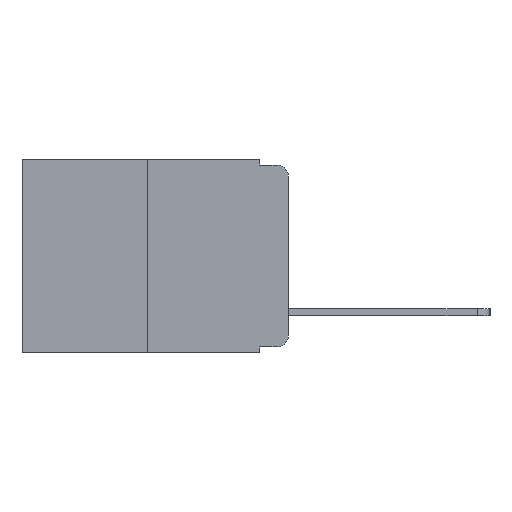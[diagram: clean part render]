
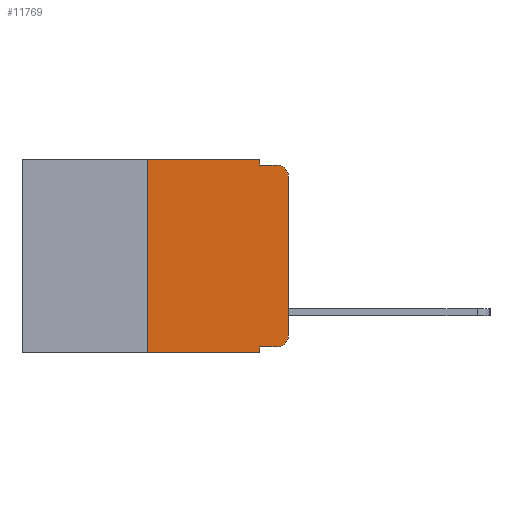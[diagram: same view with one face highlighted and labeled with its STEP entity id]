
A CAD part, left-side view. The second image highlights one B-rep face of the part: STEP entity #11769.
In plain terms, the highlighted planar face has unit normal (-1, 0, 0).
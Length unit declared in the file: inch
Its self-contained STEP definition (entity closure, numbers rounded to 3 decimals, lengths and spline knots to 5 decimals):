
#144 = ORIENTED_EDGE ( 'NONE', *, *, #9929, .F. ) ;
#289 = EDGE_CURVE ( 'NONE', #15602, #3585, #14269, .T. ) ;
#382 = CARTESIAN_POINT ( 'NONE',  ( 0., 0., 0. ) ) ;
#450 = CARTESIAN_POINT ( 'NONE',  ( 0., 0.25, 0. ) ) ;
#465 = ORIENTED_EDGE ( 'NONE', *, *, #289, .F. ) ;
#597 = EDGE_CURVE ( 'NONE', #3585, #1337, #13686, .T. ) ;
#1115 = PLANE ( 'NONE',  #10771 ) ;
#1337 = VERTEX_POINT ( 'NONE', #8802 ) ;
#1587 = EDGE_CURVE ( 'NONE', #6925, #15602, #7060, .T. ) ;
#1869 = VECTOR ( 'NONE', #12917, 39.37008 ) ;
#1883 = AXIS2_PLACEMENT_3D ( 'NONE', #12427, #4778, #13621 ) ;
#1904 = CARTESIAN_POINT ( 'NONE',  ( 0., 0.051, 0. ) ) ;
#1936 = EDGE_CURVE ( 'NONE', #15702, #2040, #3528, .T. ) ;
#2040 = VERTEX_POINT ( 'NONE', #13133 ) ;
#2333 = ORIENTED_EDGE ( 'NONE', *, *, #15019, .T. ) ;
#2790 = CARTESIAN_POINT ( 'NONE',  ( 0., 0.051, -0.333 ) ) ;
#2798 = ORIENTED_EDGE ( 'NONE', *, *, #3509, .F. ) ;
#3170 = DIRECTION ( 'NONE',  ( 0., -1., 0. ) ) ;
#3424 = ORIENTED_EDGE ( 'NONE', *, *, #1587, .F. ) ;
#3509 = EDGE_CURVE ( 'NONE', #9768, #4463, #15355, .T. ) ;
#3528 = LINE ( 'NONE', #382, #13661 ) ;
#3548 = CARTESIAN_POINT ( 'NONE',  ( 0., 0.051, 0. ) ) ;
#3585 = VERTEX_POINT ( 'NONE', #13526 ) ;
#3681 = CARTESIAN_POINT ( 'NONE',  ( 0., 0.25, 0. ) ) ;
#3753 = CARTESIAN_POINT ( 'NONE',  ( 0., 0.25, -0.343 ) ) ;
#3806 = VERTEX_POINT ( 'NONE', #15299 ) ;
#4184 = FACE_OUTER_BOUND ( 'NONE', #12924, .T. ) ;
#4307 = DIRECTION ( 'NONE',  ( 0., 0., 1. ) ) ;
#4463 = VERTEX_POINT ( 'NONE', #14664 ) ;
#4642 = LINE ( 'NONE', #15768, #15094 ) ;
#4778 = DIRECTION ( 'NONE',  ( -1., 0., 0. ) ) ;
#4926 = CARTESIAN_POINT ( 'NONE',  ( 0., 0.02, -0.333 ) ) ;
#5061 = VECTOR ( 'NONE', #3170, 39.37008 ) ;
#5252 = EDGE_CURVE ( 'NONE', #9768, #7933, #14717, .T. ) ;
#5268 = DIRECTION ( 'NONE',  ( 1., 0., 0. ) ) ;
#5743 = VECTOR ( 'NONE', #13555, 39.37008 ) ;
#6123 = EDGE_CURVE ( 'NONE', #7933, #15702, #8132, .T. ) ;
#6925 = VERTEX_POINT ( 'NONE', #3753 ) ;
#7060 = LINE ( 'NONE', #450, #13671 ) ;
#7071 = VECTOR ( 'NONE', #10058, 39.37008 ) ;
#7110 = DIRECTION ( 'NONE',  ( 0., -1., 0. ) ) ;
#7153 = DIRECTION ( 'NONE',  ( 0., -1., 0. ) ) ;
#7773 = CARTESIAN_POINT ( 'NONE',  ( 0., 0.473, 0. ) ) ;
#7933 = VERTEX_POINT ( 'NONE', #4926 ) ;
#8132 = CIRCLE ( 'NONE', #15041, 0.02 ) ;
#8161 = ORIENTED_EDGE ( 'NONE', *, *, #5252, .T. ) ;
#8312 = ORIENTED_EDGE ( 'NONE', *, *, #6123, .T. ) ;
#8504 = ORIENTED_EDGE ( 'NONE', *, *, #9067, .T. ) ;
#8802 = CARTESIAN_POINT ( 'NONE',  ( 0., 0.051, -0.01 ) ) ;
#8965 = LINE ( 'NONE', #16425, #1869 ) ;
#9067 = EDGE_CURVE ( 'NONE', #2040, #3806, #10832, .T. ) ;
#9768 = VERTEX_POINT ( 'NONE', #2790 ) ;
#9929 = EDGE_CURVE ( 'NONE', #1337, #3806, #4642, .T. ) ;
#10058 = DIRECTION ( 'NONE',  ( 0., 0., -1. ) ) ;
#10247 = DIRECTION ( 'NONE',  ( -1., 0., 0. ) ) ;
#10416 = DIRECTION ( 'NONE',  ( 0., 0., -1. ) ) ;
#10681 = VECTOR ( 'NONE', #7153, 39.37008 ) ;
#10771 = AXIS2_PLACEMENT_3D ( 'NONE', #12892, #5268, #14085 ) ;
#10832 = CIRCLE ( 'NONE', #1883, 0.02 ) ;
#10933 = CARTESIAN_POINT ( 'NONE',  ( 0., 0.02, -0.313 ) ) ;
#11633 = ORIENTED_EDGE ( 'NONE', *, *, #597, .F. ) ;
#11769 = ADVANCED_FACE ( 'NONE', ( #4184 ), #1115, .F. ) ;
#12427 = CARTESIAN_POINT ( 'NONE',  ( 0., 0.02, -0.03 ) ) ;
#12892 = CARTESIAN_POINT ( 'NONE',  ( 0., 0.473, 0. ) ) ;
#12917 = DIRECTION ( 'NONE',  ( 0., -1., 0. ) ) ;
#12924 = EDGE_LOOP ( 'NONE', ( #13940, #8504, #144, #11633, #465, #3424, #2333, #2798, #8161, #8312 ) ) ;
#12997 = DIRECTION ( 'NONE',  ( 0., 0., 1. ) ) ;
#13021 = CARTESIAN_POINT ( 'NONE',  ( 0., 0., -0.313 ) ) ;
#13133 = CARTESIAN_POINT ( 'NONE',  ( 0., 0., -0.03 ) ) ;
#13526 = CARTESIAN_POINT ( 'NONE',  ( 0., 0.051, 0. ) ) ;
#13555 = DIRECTION ( 'NONE',  ( 0., 0., -1. ) ) ;
#13621 = DIRECTION ( 'NONE',  ( 0., 0., -1. ) ) ;
#13661 = VECTOR ( 'NONE', #12997, 39.37008 ) ;
#13671 = VECTOR ( 'NONE', #4307, 39.37008 ) ;
#13686 = LINE ( 'NONE', #3548, #7071 ) ;
#13940 = ORIENTED_EDGE ( 'NONE', *, *, #1936, .T. ) ;
#14085 = DIRECTION ( 'NONE',  ( 0., 0., -1. ) ) ;
#14269 = LINE ( 'NONE', #7773, #10681 ) ;
#14664 = CARTESIAN_POINT ( 'NONE',  ( 0., 0.051, -0.343 ) ) ;
#14717 = LINE ( 'NONE', #14980, #5061 ) ;
#14980 = CARTESIAN_POINT ( 'NONE',  ( 0., 0.051, -0.333 ) ) ;
#15019 = EDGE_CURVE ( 'NONE', #6925, #4463, #8965, .T. ) ;
#15041 = AXIS2_PLACEMENT_3D ( 'NONE', #10933, #10247, #10416 ) ;
#15094 = VECTOR ( 'NONE', #7110, 39.37008 ) ;
#15299 = CARTESIAN_POINT ( 'NONE',  ( 0., 0.02, -0.01 ) ) ;
#15355 = LINE ( 'NONE', #1904, #5743 ) ;
#15602 = VERTEX_POINT ( 'NONE', #3681 ) ;
#15702 = VERTEX_POINT ( 'NONE', #13021 ) ;
#15768 = CARTESIAN_POINT ( 'NONE',  ( 0., 0.051, -0.01 ) ) ;
#16425 = CARTESIAN_POINT ( 'NONE',  ( 0., 0.473, -0.343 ) ) ;
